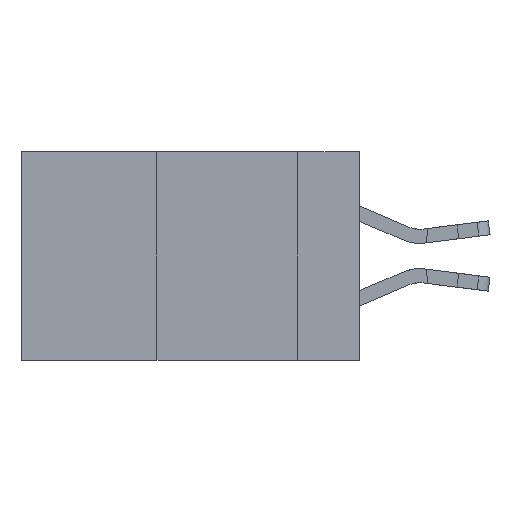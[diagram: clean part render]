
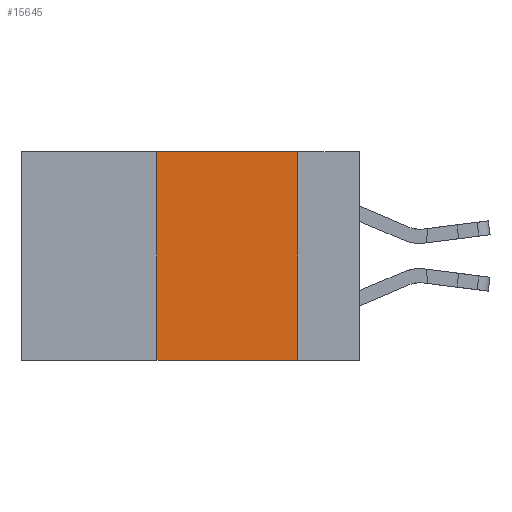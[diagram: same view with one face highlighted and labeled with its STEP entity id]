
A CAD part, left-side view. The second image highlights one B-rep face of the part: STEP entity #15645.
In plain terms, the highlighted planar face has unit normal (-1, 0, 0).
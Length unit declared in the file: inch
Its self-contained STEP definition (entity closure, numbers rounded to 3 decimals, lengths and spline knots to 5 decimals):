
#557 = CARTESIAN_POINT ( 'NONE',  ( 0., 0.11, 0. ) ) ;
#1017 = LINE ( 'NONE', #15513, #25437 ) ;
#1163 = ORIENTED_EDGE ( 'NONE', *, *, #18178, .F. ) ;
#2998 = EDGE_CURVE ( 'NONE', #9932, #14371, #21931, .T. ) ;
#3619 = ORIENTED_EDGE ( 'NONE', *, *, #16715, .F. ) ;
#3931 = CARTESIAN_POINT ( 'NONE',  ( 0., 0.36, -0.37 ) ) ;
#6759 = CARTESIAN_POINT ( 'NONE',  ( 0., 0.11, -0.37 ) ) ;
#6911 = CARTESIAN_POINT ( 'NONE',  ( 0., 0.6, 0. ) ) ;
#9095 = ORIENTED_EDGE ( 'NONE', *, *, #13111, .F. ) ;
#9285 = VERTEX_POINT ( 'NONE', #13338 ) ;
#9932 = VERTEX_POINT ( 'NONE', #3931 ) ;
#10362 = CARTESIAN_POINT ( 'NONE',  ( 0., 0.6, 0. ) ) ;
#10860 = LINE ( 'NONE', #6911, #21839 ) ;
#11385 = VECTOR ( 'NONE', #19952, 39.37008 ) ;
#11910 = CARTESIAN_POINT ( 'NONE',  ( 0., 0.6, -0.37 ) ) ;
#11942 = VERTEX_POINT ( 'NONE', #21259 ) ;
#12561 = LINE ( 'NONE', #557, #23346 ) ;
#12761 = EDGE_LOOP ( 'NONE', ( #1163, #9095, #3619, #19534 ) ) ;
#13111 = EDGE_CURVE ( 'NONE', #9285, #11942, #10860, .T. ) ;
#13338 = CARTESIAN_POINT ( 'NONE',  ( 0., 0.36, 0. ) ) ;
#14196 = DIRECTION ( 'NONE',  ( 0., 0., -1. ) ) ;
#14371 = VERTEX_POINT ( 'NONE', #6759 ) ;
#15513 = CARTESIAN_POINT ( 'NONE',  ( 0., 0.36, 0. ) ) ;
#15645 = ADVANCED_FACE ( 'NONE', ( #18793 ), #16429, .F. ) ;
#16429 = PLANE ( 'NONE',  #25875 ) ;
#16715 = EDGE_CURVE ( 'NONE', #9932, #9285, #1017, .T. ) ;
#18178 = EDGE_CURVE ( 'NONE', #11942, #14371, #12561, .T. ) ;
#18793 = FACE_OUTER_BOUND ( 'NONE', #12761, .T. ) ;
#19534 = ORIENTED_EDGE ( 'NONE', *, *, #2998, .T. ) ;
#19604 = DIRECTION ( 'NONE',  ( 0., 0., 1. ) ) ;
#19952 = DIRECTION ( 'NONE',  ( 0., -1., 0. ) ) ;
#20261 = DIRECTION ( 'NONE',  ( 1., 0., 0. ) ) ;
#21259 = CARTESIAN_POINT ( 'NONE',  ( 0., 0.11, 0. ) ) ;
#21839 = VECTOR ( 'NONE', #22993, 39.37008 ) ;
#21931 = LINE ( 'NONE', #11910, #11385 ) ;
#22993 = DIRECTION ( 'NONE',  ( 0., -1., 0. ) ) ;
#23346 = VECTOR ( 'NONE', #24572, 39.37008 ) ;
#24572 = DIRECTION ( 'NONE',  ( 0., 0., -1. ) ) ;
#25437 = VECTOR ( 'NONE', #19604, 39.37008 ) ;
#25875 = AXIS2_PLACEMENT_3D ( 'NONE', #10362, #20261, #14196 ) ;
